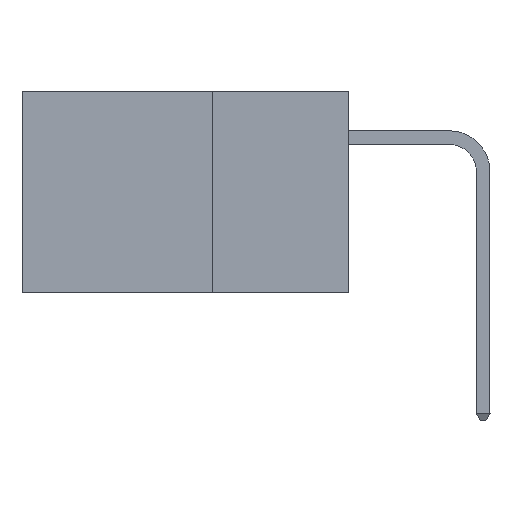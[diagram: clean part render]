
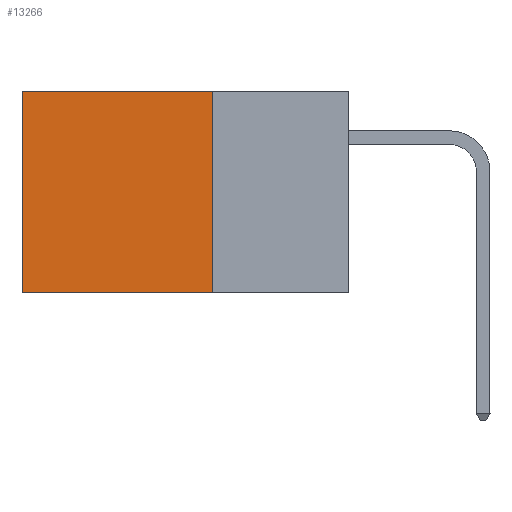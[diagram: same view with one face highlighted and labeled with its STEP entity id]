
A CAD part, left-side view. The second image highlights one B-rep face of the part: STEP entity #13266.
In plain terms, the highlighted planar face has unit normal (-1, 0, 0).
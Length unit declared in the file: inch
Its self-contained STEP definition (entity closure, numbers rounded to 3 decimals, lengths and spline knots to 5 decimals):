
#658 = VECTOR ( 'NONE', #10793, 39.37008 ) ;
#1473 = AXIS2_PLACEMENT_3D ( 'NONE', #21085, #12163, #28041 ) ;
#1904 = ORIENTED_EDGE ( 'NONE', *, *, #3940, .F. ) ;
#3940 = EDGE_CURVE ( 'NONE', #29080, #7334, #18451, .T. ) ;
#5417 = DIRECTION ( 'NONE',  ( 0., 0., -1. ) ) ;
#5477 = CARTESIAN_POINT ( 'NONE',  ( 0.2875, 0.25, -0.37 ) ) ;
#6931 = VECTOR ( 'NONE', #39716, 39.37008 ) ;
#7334 = VERTEX_POINT ( 'NONE', #20847 ) ;
#8164 = LINE ( 'NONE', #20770, #6931 ) ;
#8540 = ORIENTED_EDGE ( 'NONE', *, *, #26033, .F. ) ;
#10793 = DIRECTION ( 'NONE',  ( 0., 1., 0. ) ) ;
#11742 = VECTOR ( 'NONE', #12016, 39.37008 ) ;
#12016 = DIRECTION ( 'NONE',  ( 0., 1., 0. ) ) ;
#12163 = DIRECTION ( 'NONE',  ( 1., 0., 0. ) ) ;
#12407 = EDGE_LOOP ( 'NONE', ( #29261, #1904, #8540, #20705 ) ) ;
#13266 = ADVANCED_FACE ( 'NONE', ( #40432 ), #14670, .F. ) ;
#14670 = PLANE ( 'NONE',  #1473 ) ;
#17047 = CARTESIAN_POINT ( 'NONE',  ( 0.2875, 0.6, 0. ) ) ;
#18451 = LINE ( 'NONE', #25015, #11742 ) ;
#20705 = ORIENTED_EDGE ( 'NONE', *, *, #36934, .T. ) ;
#20770 = CARTESIAN_POINT ( 'NONE',  ( 0.2875, 0.25, 0. ) ) ;
#20847 = CARTESIAN_POINT ( 'NONE',  ( 0.2875, 0.6, -0.37 ) ) ;
#21085 = CARTESIAN_POINT ( 'NONE',  ( 0.2875, 0.25, 0. ) ) ;
#21603 = VECTOR ( 'NONE', #5417, 39.37008 ) ;
#25015 = CARTESIAN_POINT ( 'NONE',  ( 0.2875, 0.25, -0.37 ) ) ;
#26033 = EDGE_CURVE ( 'NONE', #38957, #29080, #8164, .T. ) ;
#26471 = CARTESIAN_POINT ( 'NONE',  ( 0.2875, 0.25, 0. ) ) ;
#28041 = DIRECTION ( 'NONE',  ( 0., 0., -1. ) ) ;
#29080 = VERTEX_POINT ( 'NONE', #5477 ) ;
#29261 = ORIENTED_EDGE ( 'NONE', *, *, #39724, .T. ) ;
#33479 = CARTESIAN_POINT ( 'NONE',  ( 0.2875, 0.6, 0. ) ) ;
#33804 = CARTESIAN_POINT ( 'NONE',  ( 0.2875, 0.25, 0. ) ) ;
#33995 = VERTEX_POINT ( 'NONE', #17047 ) ;
#36934 = EDGE_CURVE ( 'NONE', #38957, #33995, #38443, .T. ) ;
#38443 = LINE ( 'NONE', #26471, #658 ) ;
#38957 = VERTEX_POINT ( 'NONE', #33804 ) ;
#39716 = DIRECTION ( 'NONE',  ( 0., 0., -1. ) ) ;
#39724 = EDGE_CURVE ( 'NONE', #33995, #7334, #40283, .T. ) ;
#40283 = LINE ( 'NONE', #33479, #21603 ) ;
#40432 = FACE_OUTER_BOUND ( 'NONE', #12407, .T. ) ;
